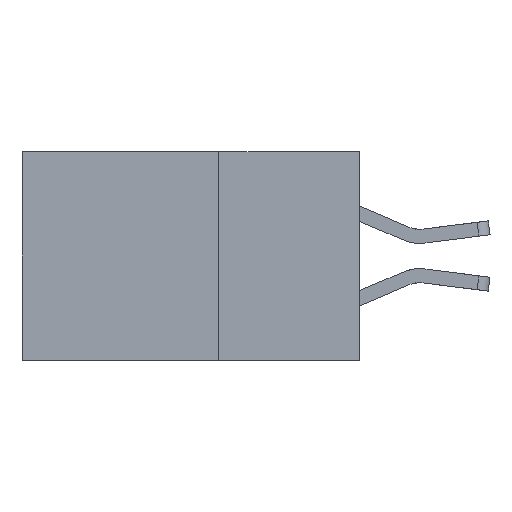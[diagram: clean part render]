
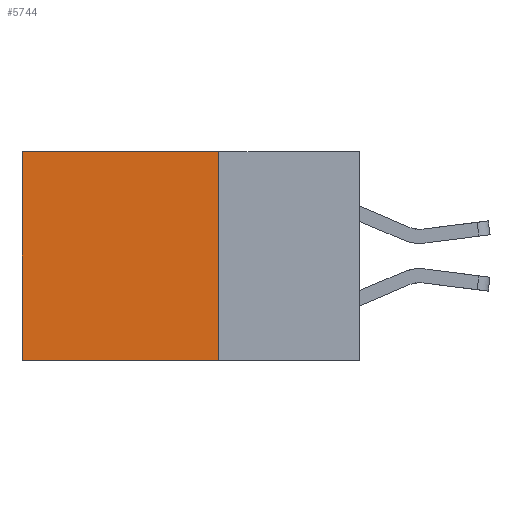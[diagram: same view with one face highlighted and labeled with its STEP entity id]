
A CAD part, left-side view. The second image highlights one B-rep face of the part: STEP entity #5744.
In plain terms, the highlighted planar face has unit normal (-1, 0, 0).
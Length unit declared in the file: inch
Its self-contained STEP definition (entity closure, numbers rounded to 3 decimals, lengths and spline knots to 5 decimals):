
#289 = EDGE_LOOP ( 'NONE', ( #14474, #8272, #2051, #3459 ) ) ;
#1078 = CARTESIAN_POINT ( 'NONE',  ( 0.2875, 0.25, -0.37 ) ) ;
#1166 = CARTESIAN_POINT ( 'NONE',  ( 0.2875, 0.25, 0. ) ) ;
#1241 = DIRECTION ( 'NONE',  ( 0., 1., 0. ) ) ;
#1250 = VECTOR ( 'NONE', #1481, 39.37008 ) ;
#1481 = DIRECTION ( 'NONE',  ( 0., 0., -1. ) ) ;
#1494 = CARTESIAN_POINT ( 'NONE',  ( 0.2875, 0.6, -0.37 ) ) ;
#1589 = EDGE_CURVE ( 'NONE', #7613, #4301, #9865, .T. ) ;
#2051 = ORIENTED_EDGE ( 'NONE', *, *, #4506, .F. ) ;
#2058 = DIRECTION ( 'NONE',  ( 0., 0., -1. ) ) ;
#2059 = CARTESIAN_POINT ( 'NONE',  ( 0.2875, 0.25, 0. ) ) ;
#2597 = VERTEX_POINT ( 'NONE', #2059 ) ;
#3097 = LINE ( 'NONE', #13783, #13578 ) ;
#3230 = FACE_OUTER_BOUND ( 'NONE', #289, .T. ) ;
#3459 = ORIENTED_EDGE ( 'NONE', *, *, #5092, .T. ) ;
#4301 = VERTEX_POINT ( 'NONE', #1494 ) ;
#4506 = EDGE_CURVE ( 'NONE', #2597, #15118, #5949, .T. ) ;
#5092 = EDGE_CURVE ( 'NONE', #2597, #7613, #3097, .T. ) ;
#5612 = DIRECTION ( 'NONE',  ( 0., 1., 0. ) ) ;
#5744 = ADVANCED_FACE ( 'NONE', ( #3230 ), #11843, .F. ) ;
#5949 = LINE ( 'NONE', #1166, #10027 ) ;
#7143 = DIRECTION ( 'NONE',  ( 1., 0., 0. ) ) ;
#7613 = VERTEX_POINT ( 'NONE', #13336 ) ;
#8272 = ORIENTED_EDGE ( 'NONE', *, *, #15061, .F. ) ;
#8550 = AXIS2_PLACEMENT_3D ( 'NONE', #9341, #7143, #2058 ) ;
#9341 = CARTESIAN_POINT ( 'NONE',  ( 0.2875, 0.25, 0. ) ) ;
#9865 = LINE ( 'NONE', #10013, #1250 ) ;
#10013 = CARTESIAN_POINT ( 'NONE',  ( 0.2875, 0.6, 0. ) ) ;
#10027 = VECTOR ( 'NONE', #13086, 39.37008 ) ;
#10890 = LINE ( 'NONE', #1078, #15021 ) ;
#11843 = PLANE ( 'NONE',  #8550 ) ;
#13086 = DIRECTION ( 'NONE',  ( 0., 0., -1. ) ) ;
#13336 = CARTESIAN_POINT ( 'NONE',  ( 0.2875, 0.6, 0. ) ) ;
#13578 = VECTOR ( 'NONE', #5612, 39.37008 ) ;
#13783 = CARTESIAN_POINT ( 'NONE',  ( 0.2875, 0.25, 0. ) ) ;
#14285 = CARTESIAN_POINT ( 'NONE',  ( 0.2875, 0.25, -0.37 ) ) ;
#14474 = ORIENTED_EDGE ( 'NONE', *, *, #1589, .T. ) ;
#15021 = VECTOR ( 'NONE', #1241, 39.37008 ) ;
#15061 = EDGE_CURVE ( 'NONE', #15118, #4301, #10890, .T. ) ;
#15118 = VERTEX_POINT ( 'NONE', #14285 ) ;
